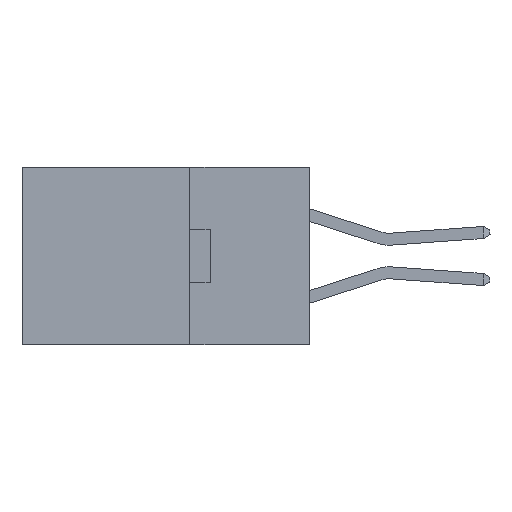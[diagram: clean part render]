
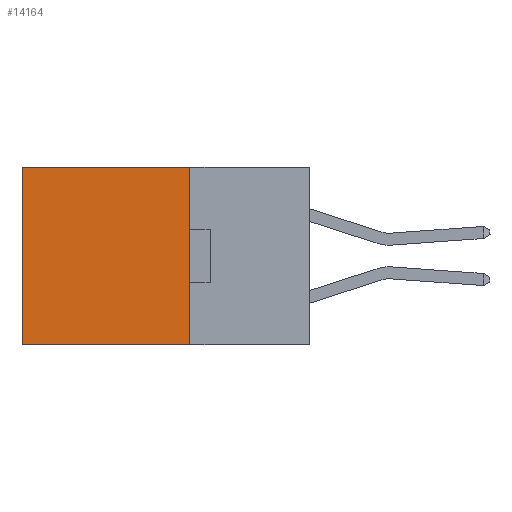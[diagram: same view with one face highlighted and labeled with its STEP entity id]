
A CAD part, left-side view. The second image highlights one B-rep face of the part: STEP entity #14164.
In plain terms, the highlighted planar face has unit normal (-1, 0, 0).
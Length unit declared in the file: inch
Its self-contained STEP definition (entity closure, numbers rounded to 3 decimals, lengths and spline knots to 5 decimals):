
#575 = EDGE_CURVE ( 'NONE', #12905, #13744, #4184, .T. ) ;
#1017 = VECTOR ( 'NONE', #14256, 39.37008 ) ;
#1191 = FACE_OUTER_BOUND ( 'NONE', #18402, .T. ) ;
#1303 = LINE ( 'NONE', #19208, #12841 ) ;
#1631 = VECTOR ( 'NONE', #24783, 39.37008 ) ;
#3478 = DIRECTION ( 'NONE',  ( 1., 0., 0. ) ) ;
#3812 = ORIENTED_EDGE ( 'NONE', *, *, #12061, .F. ) ;
#4184 = LINE ( 'NONE', #23701, #10172 ) ;
#4490 = EDGE_CURVE ( 'NONE', #15306, #21033, #16166, .T. ) ;
#7941 = LINE ( 'NONE', #24892, #1017 ) ;
#8369 = CARTESIAN_POINT ( 'NONE',  ( 0.2615, 0.6, -0.37 ) ) ;
#9235 = CARTESIAN_POINT ( 'NONE',  ( 0.2615, 0.25, -0.37 ) ) ;
#9247 = AXIS2_PLACEMENT_3D ( 'NONE', #16681, #3478, #13970 ) ;
#10060 = DIRECTION ( 'NONE',  ( 0., 0., -1. ) ) ;
#10172 = VECTOR ( 'NONE', #12805, 39.37008 ) ;
#11261 = ORIENTED_EDGE ( 'NONE', *, *, #4490, .F. ) ;
#11586 = CARTESIAN_POINT ( 'NONE',  ( 0.2615, 0.25, -0.37 ) ) ;
#12061 = EDGE_CURVE ( 'NONE', #12905, #15306, #1303, .T. ) ;
#12805 = DIRECTION ( 'NONE',  ( 0., 1., 0. ) ) ;
#12841 = VECTOR ( 'NONE', #10060, 39.37008 ) ;
#12905 = VERTEX_POINT ( 'NONE', #27763 ) ;
#13744 = VERTEX_POINT ( 'NONE', #14424 ) ;
#13970 = DIRECTION ( 'NONE',  ( 0., 0., -1. ) ) ;
#14159 = EDGE_CURVE ( 'NONE', #13744, #21033, #7941, .T. ) ;
#14164 = ADVANCED_FACE ( 'NONE', ( #1191 ), #25026, .F. ) ;
#14256 = DIRECTION ( 'NONE',  ( 0., 0., -1. ) ) ;
#14424 = CARTESIAN_POINT ( 'NONE',  ( 0.2615, 0.6, 0. ) ) ;
#15306 = VERTEX_POINT ( 'NONE', #9235 ) ;
#15591 = ORIENTED_EDGE ( 'NONE', *, *, #575, .T. ) ;
#16166 = LINE ( 'NONE', #11586, #1631 ) ;
#16681 = CARTESIAN_POINT ( 'NONE',  ( 0.2615, 0.25, -0.37 ) ) ;
#18402 = EDGE_LOOP ( 'NONE', ( #23101, #11261, #3812, #15591 ) ) ;
#19208 = CARTESIAN_POINT ( 'NONE',  ( 0.2615, 0.25, -0.37 ) ) ;
#21033 = VERTEX_POINT ( 'NONE', #8369 ) ;
#23101 = ORIENTED_EDGE ( 'NONE', *, *, #14159, .T. ) ;
#23701 = CARTESIAN_POINT ( 'NONE',  ( 0.2615, 0.25, 0. ) ) ;
#24783 = DIRECTION ( 'NONE',  ( 0., 1., 0. ) ) ;
#24892 = CARTESIAN_POINT ( 'NONE',  ( 0.2615, 0.6, -0.37 ) ) ;
#25026 = PLANE ( 'NONE',  #9247 ) ;
#27763 = CARTESIAN_POINT ( 'NONE',  ( 0.2615, 0.25, 0. ) ) ;
